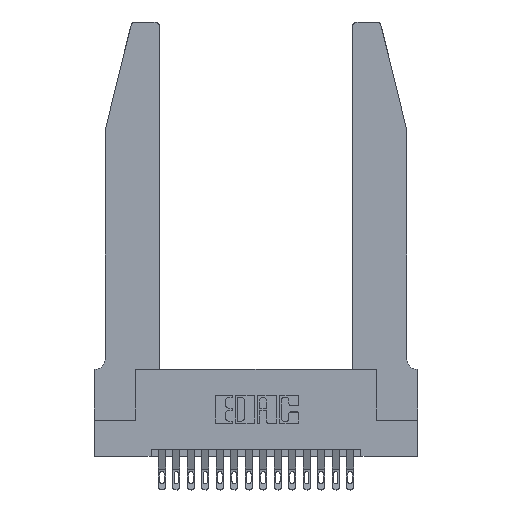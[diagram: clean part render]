
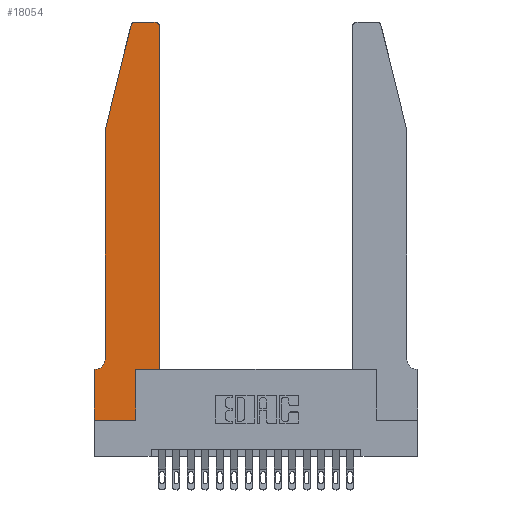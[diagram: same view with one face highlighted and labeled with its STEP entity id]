
A CAD part, top view. The second image highlights one B-rep face of the part: STEP entity #18054.
In plain terms, the highlighted planar face has unit normal (0, 0, 1).
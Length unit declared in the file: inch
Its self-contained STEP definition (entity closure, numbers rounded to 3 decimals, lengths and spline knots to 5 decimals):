
#38 = LINE ( 'NONE', #13793, #5779 ) ;
#176 = CARTESIAN_POINT ( 'NONE',  ( 0.4505, 2.72, 0.37 ) ) ;
#362 = DIRECTION ( 'NONE',  ( 0., 1., 0. ) ) ;
#857 = EDGE_CURVE ( 'NONE', #12377, #3170, #10299, .T. ) ;
#1085 = DIRECTION ( 'NONE',  ( 0., 0., 1. ) ) ;
#1143 = VERTEX_POINT ( 'NONE', #11178 ) ;
#1276 = CARTESIAN_POINT ( 'NONE',  ( 0.0055, 0.42, 0.37 ) ) ;
#1622 = EDGE_CURVE ( 'NONE', #8771, #7121, #5789, .T. ) ;
#1623 = EDGE_CURVE ( 'NONE', #2508, #12377, #16529, .T. ) ;
#2133 = VECTOR ( 'NONE', #18279, 39.37008 ) ;
#2325 = VECTOR ( 'NONE', #17702, 39.37008 ) ;
#2508 = VERTEX_POINT ( 'NONE', #13545 ) ;
#2621 = ORIENTED_EDGE ( 'NONE', *, *, #11000, .T. ) ;
#2631 = CARTESIAN_POINT ( 'NONE',  ( 0.0755, 2., 0.37 ) ) ;
#2659 = VECTOR ( 'NONE', #10802, 39.37008 ) ;
#3008 = DIRECTION ( 'NONE',  ( 0., 0., -1. ) ) ;
#3170 = VERTEX_POINT ( 'NONE', #15857 ) ;
#3548 = ORIENTED_EDGE ( 'NONE', *, *, #15578, .T. ) ;
#3586 = LINE ( 'NONE', #16979, #2659 ) ;
#3975 = DIRECTION ( 'NONE',  ( 1., 0., 0. ) ) ;
#4270 = DIRECTION ( 'NONE',  ( -1., 0., 0. ) ) ;
#4297 = ORIENTED_EDGE ( 'NONE', *, *, #18033, .T. ) ;
#4915 = EDGE_CURVE ( 'NONE', #19642, #19420, #19795, .T. ) ;
#5098 = AXIS2_PLACEMENT_3D ( 'NONE', #7178, #19463, #13404 ) ;
#5267 = VECTOR ( 'NONE', #18074, 39.37008 ) ;
#5570 = PLANE ( 'NONE',  #17865 ) ;
#5779 = VECTOR ( 'NONE', #7459, 39.37008 ) ;
#5789 = CIRCLE ( 'NONE', #5949, 0.07 ) ;
#5872 = EDGE_CURVE ( 'NONE', #14095, #1143, #17329, .T. ) ;
#5949 = AXIS2_PLACEMENT_3D ( 'NONE', #1276, #3008, #4270 ) ;
#6094 = CARTESIAN_POINT ( 'NONE',  ( 0., 0.35, 0.37 ) ) ;
#6526 = ORIENTED_EDGE ( 'NONE', *, *, #857, .T. ) ;
#6739 = CARTESIAN_POINT ( 'NONE',  ( 0.284, 2.75, 0.37 ) ) ;
#6749 = EDGE_LOOP ( 'NONE', ( #10567, #16776, #13372, #4297, #14602, #2621, #3548, #9317, #8814, #11204, #18023, #6526 ) ) ;
#7107 = CARTESIAN_POINT ( 'NONE',  ( 0., 0.35, 0.37 ) ) ;
#7121 = VERTEX_POINT ( 'NONE', #18173 ) ;
#7178 = CARTESIAN_POINT ( 'NONE',  ( 0.284, 2.72, 0.37 ) ) ;
#7317 = LINE ( 'NONE', #14288, #18831 ) ;
#7359 = FACE_OUTER_BOUND ( 'NONE', #6749, .T. ) ;
#7458 = AXIS2_PLACEMENT_3D ( 'NONE', #19344, #16169, #3975 ) ;
#7459 = DIRECTION ( 'NONE',  ( 0., -1., 0. ) ) ;
#7569 = EDGE_CURVE ( 'NONE', #18205, #14095, #13185, .T. ) ;
#7627 = EDGE_CURVE ( 'NONE', #3170, #19642, #3586, .T. ) ;
#7674 = DIRECTION ( 'NONE',  ( -1., 0., 0. ) ) ;
#8457 = VERTEX_POINT ( 'NONE', #12339 ) ;
#8712 = CARTESIAN_POINT ( 'NONE',  ( 0.0755, 0.35, 0.37 ) ) ;
#8771 = VERTEX_POINT ( 'NONE', #12808 ) ;
#8814 = ORIENTED_EDGE ( 'NONE', *, *, #5872, .T. ) ;
#9086 = CARTESIAN_POINT ( 'NONE',  ( 0.4505, 0.35, 0.37 ) ) ;
#9228 = LINE ( 'NONE', #8712, #11345 ) ;
#9317 = ORIENTED_EDGE ( 'NONE', *, *, #7569, .T. ) ;
#10039 = DIRECTION ( 'NONE',  ( 1., 0., 0. ) ) ;
#10299 = CIRCLE ( 'NONE', #7458, 0.03 ) ;
#10481 = DIRECTION ( 'NONE',  ( 0., 1., 0. ) ) ;
#10567 = ORIENTED_EDGE ( 'NONE', *, *, #7627, .T. ) ;
#10802 = DIRECTION ( 'NONE',  ( -1., 0., 0. ) ) ;
#11000 = EDGE_CURVE ( 'NONE', #7121, #16955, #9228, .T. ) ;
#11126 = EDGE_CURVE ( 'NONE', #1143, #2508, #7317, .T. ) ;
#11178 = CARTESIAN_POINT ( 'NONE',  ( 0.2865, 0.35, 0.37 ) ) ;
#11204 = ORIENTED_EDGE ( 'NONE', *, *, #11126, .T. ) ;
#11345 = VECTOR ( 'NONE', #7674, 39.37008 ) ;
#11397 = LINE ( 'NONE', #2631, #2325 ) ;
#11936 = CARTESIAN_POINT ( 'NONE',  ( 0.25487, 2.72718, 0.37 ) ) ;
#12339 = CARTESIAN_POINT ( 'NONE',  ( 0.0755, 2., 0.37 ) ) ;
#12377 = VERTEX_POINT ( 'NONE', #176 ) ;
#12808 = CARTESIAN_POINT ( 'NONE',  ( 0.0755, 0.42, 0.37 ) ) ;
#13185 = LINE ( 'NONE', #16523, #5267 ) ;
#13372 = ORIENTED_EDGE ( 'NONE', *, *, #16897, .T. ) ;
#13393 = LINE ( 'NONE', #18215, #2133 ) ;
#13404 = DIRECTION ( 'NONE',  ( 1., 0., 0. ) ) ;
#13545 = CARTESIAN_POINT ( 'NONE',  ( 0.4505, 0.35, 0.37 ) ) ;
#13793 = CARTESIAN_POINT ( 'NONE',  ( 0., 0., 0.37 ) ) ;
#14095 = VERTEX_POINT ( 'NONE', #18833 ) ;
#14272 = CARTESIAN_POINT ( 'NONE',  ( 0.2865, 0.35, 0.37 ) ) ;
#14288 = CARTESIAN_POINT ( 'NONE',  ( 0.4505, 0.35, 0.37 ) ) ;
#14602 = ORIENTED_EDGE ( 'NONE', *, *, #1622, .T. ) ;
#15577 = VECTOR ( 'NONE', #10481, 39.37008 ) ;
#15578 = EDGE_CURVE ( 'NONE', #16955, #18205, #38, .T. ) ;
#15857 = CARTESIAN_POINT ( 'NONE',  ( 0.4205, 2.75, 0.37 ) ) ;
#16169 = DIRECTION ( 'NONE',  ( 0., 0., 1. ) ) ;
#16523 = CARTESIAN_POINT ( 'NONE',  ( 0., 0., 0.37 ) ) ;
#16529 = LINE ( 'NONE', #9086, #15577 ) ;
#16776 = ORIENTED_EDGE ( 'NONE', *, *, #4915, .T. ) ;
#16858 = VECTOR ( 'NONE', #362, 39.37008 ) ;
#16897 = EDGE_CURVE ( 'NONE', #19420, #8457, #13393, .T. ) ;
#16955 = VERTEX_POINT ( 'NONE', #6094 ) ;
#16979 = CARTESIAN_POINT ( 'NONE',  ( 0.2605, 2.75, 0.37 ) ) ;
#17329 = LINE ( 'NONE', #14272, #16858 ) ;
#17702 = DIRECTION ( 'NONE',  ( 0., -1., 0. ) ) ;
#17857 = DIRECTION ( 'NONE',  ( 1., 0., 0. ) ) ;
#17865 = AXIS2_PLACEMENT_3D ( 'NONE', #7107, #1085, #10039 ) ;
#18023 = ORIENTED_EDGE ( 'NONE', *, *, #1623, .T. ) ;
#18033 = EDGE_CURVE ( 'NONE', #8457, #8771, #11397, .T. ) ;
#18054 = ADVANCED_FACE ( 'NONE', ( #7359 ), #5570, .T. ) ;
#18074 = DIRECTION ( 'NONE',  ( 1., 0., 0. ) ) ;
#18173 = CARTESIAN_POINT ( 'NONE',  ( 0.0055, 0.35, 0.37 ) ) ;
#18205 = VERTEX_POINT ( 'NONE', #19708 ) ;
#18215 = CARTESIAN_POINT ( 'NONE',  ( 0.0755, 2., 0.37 ) ) ;
#18279 = DIRECTION ( 'NONE',  ( -0.239, -0.971, 0. ) ) ;
#18831 = VECTOR ( 'NONE', #17857, 39.37008 ) ;
#18833 = CARTESIAN_POINT ( 'NONE',  ( 0.2865, 0., 0.37 ) ) ;
#19344 = CARTESIAN_POINT ( 'NONE',  ( 0.4205, 2.72, 0.37 ) ) ;
#19420 = VERTEX_POINT ( 'NONE', #11936 ) ;
#19463 = DIRECTION ( 'NONE',  ( 0., 0., 1. ) ) ;
#19642 = VERTEX_POINT ( 'NONE', #6739 ) ;
#19708 = CARTESIAN_POINT ( 'NONE',  ( 0., 0., 0.37 ) ) ;
#19795 = CIRCLE ( 'NONE', #5098, 0.03 ) ;
